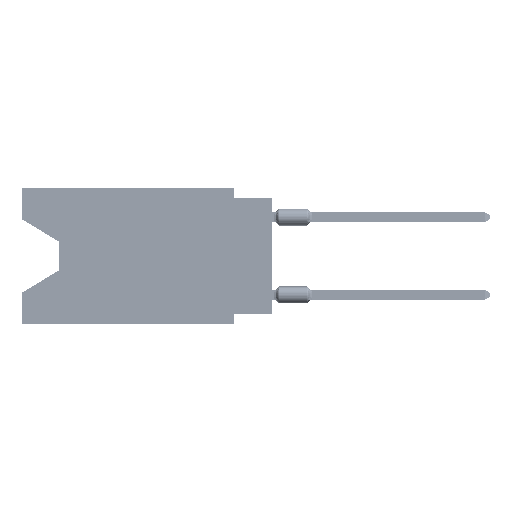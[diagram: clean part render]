
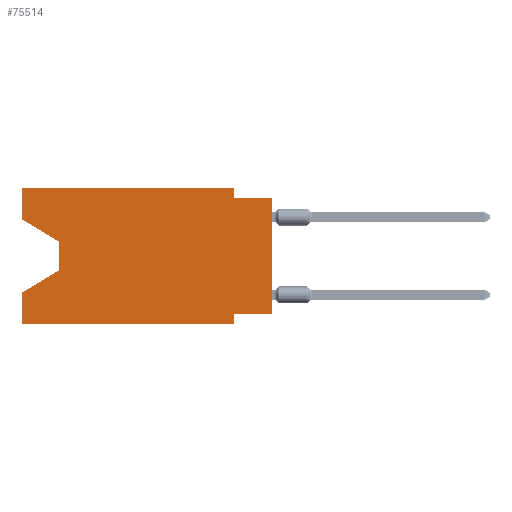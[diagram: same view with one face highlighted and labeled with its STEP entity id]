
A CAD part, left-side view. The second image highlights one B-rep face of the part: STEP entity #75514.
In plain terms, the highlighted planar face has unit normal (-1, 0, 0).
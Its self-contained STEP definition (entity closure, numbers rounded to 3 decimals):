
#314 = CARTESIAN_POINT ( 'NONE',  ( 0., 0., 0. ) ) ;
#1009 = LINE ( 'NONE', #24741, #9486 ) ;
#1881 = VECTOR ( 'NONE', #4134, 1000. ) ;
#4134 = DIRECTION ( 'NONE',  ( 0., -1., 0. ) ) ;
#4713 = VECTOR ( 'NONE', #45153, 1000. ) ;
#5349 = ORIENTED_EDGE ( 'NONE', *, *, #53135, .F. ) ;
#5778 = EDGE_CURVE ( 'NONE', #23587, #50524, #62980, .T. ) ;
#6492 = VECTOR ( 'NONE', #56319, 1000. ) ;
#7290 = ORIENTED_EDGE ( 'NONE', *, *, #22606, .F. ) ;
#7662 = LINE ( 'NONE', #31401, #76076 ) ;
#9134 = EDGE_CURVE ( 'NONE', #73452, #65365, #9959, .T. ) ;
#9410 = CARTESIAN_POINT ( 'NONE',  ( 0., 2.54, -8.89 ) ) ;
#9486 = VECTOR ( 'NONE', #65223, 1000. ) ;
#9671 = CARTESIAN_POINT ( 'NONE',  ( 0., 16.383, 0. ) ) ;
#9959 = LINE ( 'NONE', #22399, #1881 ) ;
#11886 = CARTESIAN_POINT ( 'NONE',  ( 0., 16.383, -2.038 ) ) ;
#12202 = EDGE_CURVE ( 'NONE', #76645, #54357, #15195, .T. ) ;
#13239 = DIRECTION ( 'NONE',  ( 0., 0., -1. ) ) ;
#15195 = LINE ( 'NONE', #38923, #4713 ) ;
#15366 = CARTESIAN_POINT ( 'NONE',  ( 0., 16.383, 0. ) ) ;
#15619 = VERTEX_POINT ( 'NONE', #57674 ) ;
#15713 = CARTESIAN_POINT ( 'NONE',  ( 0., 2.54, 0. ) ) ;
#15862 = ORIENTED_EDGE ( 'NONE', *, *, #36716, .T. ) ;
#15928 = DIRECTION ( 'NONE',  ( 0., 0., -1. ) ) ;
#17192 = DIRECTION ( 'NONE',  ( 0., 0., 1. ) ) ;
#17330 = ORIENTED_EDGE ( 'NONE', *, *, #34637, .F. ) ;
#19585 = CARTESIAN_POINT ( 'NONE',  ( 0., 13.97, -5.385 ) ) ;
#19692 = CARTESIAN_POINT ( 'NONE',  ( 0., 0., -8.255 ) ) ;
#19767 = DIRECTION ( 'NONE',  ( 0., -1., 0. ) ) ;
#20813 = VERTEX_POINT ( 'NONE', #29063 ) ;
#22198 = ORIENTED_EDGE ( 'NONE', *, *, #61995, .T. ) ;
#22399 = CARTESIAN_POINT ( 'NONE',  ( 0., 16.383, 0. ) ) ;
#22606 = EDGE_CURVE ( 'NONE', #72741, #29685, #24824, .T. ) ;
#23587 = VERTEX_POINT ( 'NONE', #19585 ) ;
#23843 = ORIENTED_EDGE ( 'NONE', *, *, #56993, .F. ) ;
#24219 = VERTEX_POINT ( 'NONE', #19692 ) ;
#24615 = VECTOR ( 'NONE', #13239, 1000. ) ;
#24741 = CARTESIAN_POINT ( 'NONE',  ( 0., 16.383, -2.038 ) ) ;
#24824 = LINE ( 'NONE', #25978, #43715 ) ;
#25978 = CARTESIAN_POINT ( 'NONE',  ( 0., 0., -0.635 ) ) ;
#27517 = EDGE_CURVE ( 'NONE', #24219, #20813, #62154, .T. ) ;
#28890 = CARTESIAN_POINT ( 'NONE',  ( 0., 0., -0.635 ) ) ;
#29063 = CARTESIAN_POINT ( 'NONE',  ( 0., 2.54, -8.255 ) ) ;
#29100 = AXIS2_PLACEMENT_3D ( 'NONE', #50951, #70383, #15928 ) ;
#29685 = VERTEX_POINT ( 'NONE', #28890 ) ;
#31401 = CARTESIAN_POINT ( 'NONE',  ( 0., 16.383, 0. ) ) ;
#32576 = VECTOR ( 'NONE', #38097, 1000. ) ;
#32588 = CARTESIAN_POINT ( 'NONE',  ( 0., 0., -8.255 ) ) ;
#34637 = EDGE_CURVE ( 'NONE', #65365, #72741, #54487, .T. ) ;
#35941 = DIRECTION ( 'NONE',  ( 0., 0., -1. ) ) ;
#36716 = EDGE_CURVE ( 'NONE', #71380, #15619, #1009, .T. ) ;
#36946 = LINE ( 'NONE', #43942, #72369 ) ;
#37405 = EDGE_LOOP ( 'NONE', ( #15862, #63995, #61809, #23843, #46833, #59028, #49573, #22198, #7290, #17330, #42064, #5349 ) ) ;
#37716 = DIRECTION ( 'NONE',  ( 0., 0., -1. ) ) ;
#38097 = DIRECTION ( 'NONE',  ( 0., 0.855, -0.519 ) ) ;
#38923 = CARTESIAN_POINT ( 'NONE',  ( 0., 16.383, -8.89 ) ) ;
#41022 = CARTESIAN_POINT ( 'NONE',  ( 0., 2.54, -8.89 ) ) ;
#41125 = EDGE_CURVE ( 'NONE', #20813, #54357, #65522, .T. ) ;
#41955 = DIRECTION ( 'NONE',  ( 0., 0., 1. ) ) ;
#42064 = ORIENTED_EDGE ( 'NONE', *, *, #9134, .F. ) ;
#43715 = VECTOR ( 'NONE', #19767, 1000. ) ;
#43942 = CARTESIAN_POINT ( 'NONE',  ( 0., 13.97, -3.505 ) ) ;
#45153 = DIRECTION ( 'NONE',  ( 0., -1., 0. ) ) ;
#46833 = ORIENTED_EDGE ( 'NONE', *, *, #12202, .T. ) ;
#49573 = ORIENTED_EDGE ( 'NONE', *, *, #27517, .F. ) ;
#50524 = VERTEX_POINT ( 'NONE', #60067 ) ;
#50951 = CARTESIAN_POINT ( 'NONE',  ( 0., 16.383, 0. ) ) ;
#52493 = FACE_OUTER_BOUND ( 'NONE', #37405, .T. ) ;
#53135 = EDGE_CURVE ( 'NONE', #71380, #73452, #7662, .T. ) ;
#53302 = VECTOR ( 'NONE', #41955, 1000. ) ;
#53619 = LINE ( 'NONE', #314, #53302 ) ;
#54010 = VECTOR ( 'NONE', #17192, 1000. ) ;
#54352 = DIRECTION ( 'NONE',  ( 0., 0., 1. ) ) ;
#54357 = VERTEX_POINT ( 'NONE', #9410 ) ;
#54487 = LINE ( 'NONE', #72377, #24615 ) ;
#56319 = DIRECTION ( 'NONE',  ( 0., 1., 0. ) ) ;
#56993 = EDGE_CURVE ( 'NONE', #76645, #50524, #71270, .T. ) ;
#57674 = CARTESIAN_POINT ( 'NONE',  ( 0., 13.97, -3.505 ) ) ;
#59028 = ORIENTED_EDGE ( 'NONE', *, *, #41125, .F. ) ;
#60067 = CARTESIAN_POINT ( 'NONE',  ( 0., 16.383, -6.852 ) ) ;
#61809 = ORIENTED_EDGE ( 'NONE', *, *, #5778, .T. ) ;
#61995 = EDGE_CURVE ( 'NONE', #24219, #29685, #53619, .T. ) ;
#62154 = LINE ( 'NONE', #32588, #6492 ) ;
#62980 = LINE ( 'NONE', #74257, #32576 ) ;
#63995 = ORIENTED_EDGE ( 'NONE', *, *, #73344, .T. ) ;
#64164 = PLANE ( 'NONE',  #29100 ) ;
#65223 = DIRECTION ( 'NONE',  ( 0., -0.855, -0.519 ) ) ;
#65365 = VERTEX_POINT ( 'NONE', #15713 ) ;
#65522 = LINE ( 'NONE', #41022, #75005 ) ;
#70383 = DIRECTION ( 'NONE',  ( 1., 0., 0. ) ) ;
#71270 = LINE ( 'NONE', #15366, #54010 ) ;
#71380 = VERTEX_POINT ( 'NONE', #11886 ) ;
#72369 = VECTOR ( 'NONE', #37716, 1000. ) ;
#72377 = CARTESIAN_POINT ( 'NONE',  ( 0., 2.54, 0. ) ) ;
#72741 = VERTEX_POINT ( 'NONE', #72962 ) ;
#72962 = CARTESIAN_POINT ( 'NONE',  ( 0., 2.54, -0.635 ) ) ;
#73344 = EDGE_CURVE ( 'NONE', #15619, #23587, #36946, .T. ) ;
#73452 = VERTEX_POINT ( 'NONE', #9671 ) ;
#73931 = CARTESIAN_POINT ( 'NONE',  ( 0., 16.383, -8.89 ) ) ;
#74257 = CARTESIAN_POINT ( 'NONE',  ( 0., 13.97, -5.385 ) ) ;
#75005 = VECTOR ( 'NONE', #35941, 1000. ) ;
#75514 = ADVANCED_FACE ( 'NONE', ( #52493 ), #64164, .F. ) ;
#76076 = VECTOR ( 'NONE', #54352, 1000. ) ;
#76645 = VERTEX_POINT ( 'NONE', #73931 ) ;
